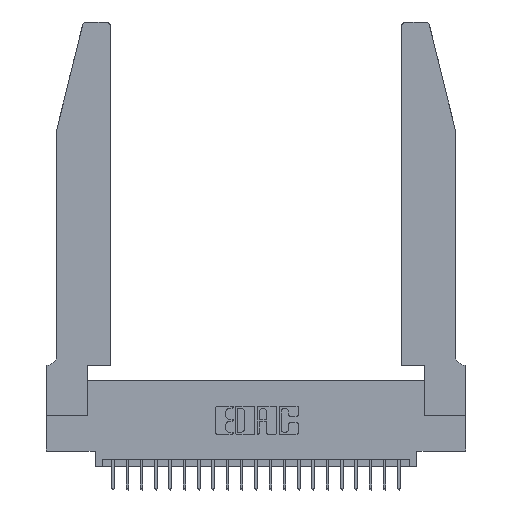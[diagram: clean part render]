
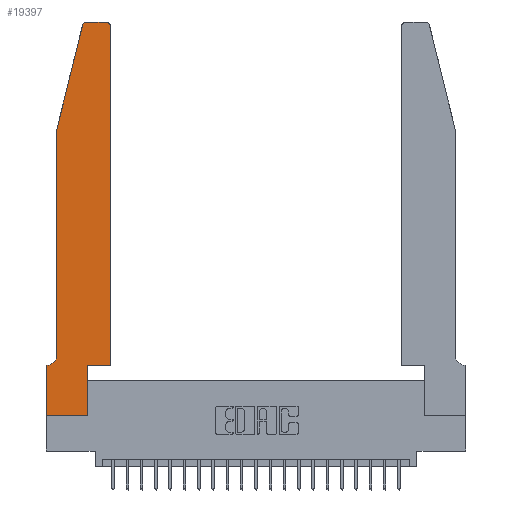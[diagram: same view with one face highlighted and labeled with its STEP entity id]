
A CAD part, top view. The second image highlights one B-rep face of the part: STEP entity #19397.
In plain terms, the highlighted planar face has unit normal (0, 0, 1).
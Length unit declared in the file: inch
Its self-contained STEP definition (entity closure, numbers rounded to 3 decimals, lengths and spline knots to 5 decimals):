
#12 = VERTEX_POINT ( 'NONE', #12040 ) ;
#38 = VERTEX_POINT ( 'NONE', #2676 ) ;
#166 = CARTESIAN_POINT ( 'NONE',  ( 0.284, 2.75, 0.37 ) ) ;
#204 = ORIENTED_EDGE ( 'NONE', *, *, #23107, .T. ) ;
#329 = LINE ( 'NONE', #17283, #21487 ) ;
#373 = CARTESIAN_POINT ( 'NONE',  ( 0.4505, 0.35, 0.37 ) ) ;
#497 = DIRECTION ( 'NONE',  ( -1., 0., 0. ) ) ;
#499 = CARTESIAN_POINT ( 'NONE',  ( 0.0755, 0.42, 0.37 ) ) ;
#772 = EDGE_CURVE ( 'NONE', #12, #782, #14708, .T. ) ;
#782 = VERTEX_POINT ( 'NONE', #8983 ) ;
#820 = ORIENTED_EDGE ( 'NONE', *, *, #18570, .T. ) ;
#1493 = CARTESIAN_POINT ( 'NONE',  ( 0.4505, 0.35, 0.37 ) ) ;
#2221 = DIRECTION ( 'NONE',  ( -0.239, -0.971, 0. ) ) ;
#2608 = CARTESIAN_POINT ( 'NONE',  ( 0.4505, 2.72, 0.37 ) ) ;
#2676 = CARTESIAN_POINT ( 'NONE',  ( 0.0055, 0.35, 0.37 ) ) ;
#3120 = DIRECTION ( 'NONE',  ( 0., 0., 1. ) ) ;
#3443 = LINE ( 'NONE', #4637, #21617 ) ;
#3552 = DIRECTION ( 'NONE',  ( 1., 0., 0. ) ) ;
#4057 = VECTOR ( 'NONE', #4981, 39.37008 ) ;
#4218 = VERTEX_POINT ( 'NONE', #22180 ) ;
#4325 = ORIENTED_EDGE ( 'NONE', *, *, #11275, .T. ) ;
#4637 = CARTESIAN_POINT ( 'NONE',  ( 0.0755, 2., 0.37 ) ) ;
#4660 = LINE ( 'NONE', #8621, #4057 ) ;
#4981 = DIRECTION ( 'NONE',  ( -1., 0., 0. ) ) ;
#5313 = ORIENTED_EDGE ( 'NONE', *, *, #23751, .T. ) ;
#5379 = EDGE_LOOP ( 'NONE', ( #23530, #5313, #16756, #22617, #18289, #8071, #4325, #22628, #17341, #204, #820, #8747 ) ) ;
#5578 = CARTESIAN_POINT ( 'NONE',  ( 0.4505, 0.35, 0.37 ) ) ;
#5833 = DIRECTION ( 'NONE',  ( 0., 0., 1. ) ) ;
#6334 = CARTESIAN_POINT ( 'NONE',  ( 0.284, 2.72, 0.37 ) ) ;
#6370 = VECTOR ( 'NONE', #9273, 39.37008 ) ;
#6829 = EDGE_CURVE ( 'NONE', #782, #18544, #11389, .T. ) ;
#6872 = CARTESIAN_POINT ( 'NONE',  ( 0., 0.35, 0.37 ) ) ;
#6983 = VECTOR ( 'NONE', #11292, 39.37008 ) ;
#7013 = CIRCLE ( 'NONE', #11297, 0.03 ) ;
#7445 = VECTOR ( 'NONE', #3552, 39.37008 ) ;
#8003 = CARTESIAN_POINT ( 'NONE',  ( 0., 0., 0.37 ) ) ;
#8071 = ORIENTED_EDGE ( 'NONE', *, *, #17658, .T. ) ;
#8502 = VERTEX_POINT ( 'NONE', #13246 ) ;
#8601 = EDGE_CURVE ( 'NONE', #4218, #18739, #329, .T. ) ;
#8621 = CARTESIAN_POINT ( 'NONE',  ( 0.0755, 0.35, 0.37 ) ) ;
#8747 = ORIENTED_EDGE ( 'NONE', *, *, #10447, .T. ) ;
#8983 = CARTESIAN_POINT ( 'NONE',  ( 0.2865, 0., 0.37 ) ) ;
#9024 = CARTESIAN_POINT ( 'NONE',  ( 0.2865, 0.35, 0.37 ) ) ;
#9054 = CARTESIAN_POINT ( 'NONE',  ( 0.0755, 2., 0.37 ) ) ;
#9273 = DIRECTION ( 'NONE',  ( 0., 1., 0. ) ) ;
#9458 = VERTEX_POINT ( 'NONE', #373 ) ;
#10409 = CARTESIAN_POINT ( 'NONE',  ( 0., 0.35, 0.37 ) ) ;
#10447 = EDGE_CURVE ( 'NONE', #21090, #4218, #7013, .T. ) ;
#10699 = AXIS2_PLACEMENT_3D ( 'NONE', #6334, #17775, #17686 ) ;
#11275 = EDGE_CURVE ( 'NONE', #18263, #12, #12577, .T. ) ;
#11292 = DIRECTION ( 'NONE',  ( 0., 1., 0. ) ) ;
#11297 = AXIS2_PLACEMENT_3D ( 'NONE', #20730, #5833, #22797 ) ;
#11385 = VERTEX_POINT ( 'NONE', #499 ) ;
#11389 = LINE ( 'NONE', #9024, #6370 ) ;
#11976 = VERTEX_POINT ( 'NONE', #12521 ) ;
#12028 = EDGE_CURVE ( 'NONE', #8502, #11976, #12811, .T. ) ;
#12040 = CARTESIAN_POINT ( 'NONE',  ( 0., 0., 0.37 ) ) ;
#12521 = CARTESIAN_POINT ( 'NONE',  ( 0.0755, 2., 0.37 ) ) ;
#12577 = LINE ( 'NONE', #8003, #19565 ) ;
#12811 = LINE ( 'NONE', #9054, #22171 ) ;
#13170 = AXIS2_PLACEMENT_3D ( 'NONE', #22550, #18770, #22481 ) ;
#13246 = CARTESIAN_POINT ( 'NONE',  ( 0.25487, 2.72718, 0.37 ) ) ;
#14624 = DIRECTION ( 'NONE',  ( 1., 0., 0. ) ) ;
#14649 = AXIS2_PLACEMENT_3D ( 'NONE', #6872, #3120, #17760 ) ;
#14708 = LINE ( 'NONE', #19689, #24085 ) ;
#16033 = PLANE ( 'NONE',  #14649 ) ;
#16756 = ORIENTED_EDGE ( 'NONE', *, *, #12028, .T. ) ;
#16931 = LINE ( 'NONE', #5578, #6983 ) ;
#17283 = CARTESIAN_POINT ( 'NONE',  ( 0.2605, 2.75, 0.37 ) ) ;
#17341 = ORIENTED_EDGE ( 'NONE', *, *, #6829, .T. ) ;
#17658 = EDGE_CURVE ( 'NONE', #38, #18263, #4660, .T. ) ;
#17686 = DIRECTION ( 'NONE',  ( 1., 0., 0. ) ) ;
#17760 = DIRECTION ( 'NONE',  ( 1., 0., 0. ) ) ;
#17775 = DIRECTION ( 'NONE',  ( 0., 0., 1. ) ) ;
#17953 = CIRCLE ( 'NONE', #10699, 0.03 ) ;
#18263 = VERTEX_POINT ( 'NONE', #10409 ) ;
#18289 = ORIENTED_EDGE ( 'NONE', *, *, #23623, .T. ) ;
#18544 = VERTEX_POINT ( 'NONE', #24025 ) ;
#18570 = EDGE_CURVE ( 'NONE', #9458, #21090, #16931, .T. ) ;
#18739 = VERTEX_POINT ( 'NONE', #166 ) ;
#18770 = DIRECTION ( 'NONE',  ( 0., 0., -1. ) ) ;
#19397 = ADVANCED_FACE ( 'NONE', ( #21604 ), #16033, .T. ) ;
#19453 = LINE ( 'NONE', #1493, #7445 ) ;
#19565 = VECTOR ( 'NONE', #22804, 39.37008 ) ;
#19689 = CARTESIAN_POINT ( 'NONE',  ( 0., 0., 0.37 ) ) ;
#20730 = CARTESIAN_POINT ( 'NONE',  ( 0.4205, 2.72, 0.37 ) ) ;
#21090 = VERTEX_POINT ( 'NONE', #2608 ) ;
#21272 = EDGE_CURVE ( 'NONE', #11976, #11385, #3443, .T. ) ;
#21487 = VECTOR ( 'NONE', #497, 39.37008 ) ;
#21604 = FACE_OUTER_BOUND ( 'NONE', #5379, .T. ) ;
#21617 = VECTOR ( 'NONE', #23579, 39.37008 ) ;
#22171 = VECTOR ( 'NONE', #2221, 39.37008 ) ;
#22180 = CARTESIAN_POINT ( 'NONE',  ( 0.4205, 2.75, 0.37 ) ) ;
#22481 = DIRECTION ( 'NONE',  ( -1., 0., 0. ) ) ;
#22550 = CARTESIAN_POINT ( 'NONE',  ( 0.0055, 0.42, 0.37 ) ) ;
#22617 = ORIENTED_EDGE ( 'NONE', *, *, #21272, .T. ) ;
#22628 = ORIENTED_EDGE ( 'NONE', *, *, #772, .T. ) ;
#22797 = DIRECTION ( 'NONE',  ( 1., 0., 0. ) ) ;
#22804 = DIRECTION ( 'NONE',  ( 0., -1., 0. ) ) ;
#23107 = EDGE_CURVE ( 'NONE', #18544, #9458, #19453, .T. ) ;
#23530 = ORIENTED_EDGE ( 'NONE', *, *, #8601, .T. ) ;
#23579 = DIRECTION ( 'NONE',  ( 0., -1., 0. ) ) ;
#23623 = EDGE_CURVE ( 'NONE', #11385, #38, #23820, .T. ) ;
#23751 = EDGE_CURVE ( 'NONE', #18739, #8502, #17953, .T. ) ;
#23820 = CIRCLE ( 'NONE', #13170, 0.07 ) ;
#24025 = CARTESIAN_POINT ( 'NONE',  ( 0.2865, 0.35, 0.37 ) ) ;
#24085 = VECTOR ( 'NONE', #14624, 39.37008 ) ;
